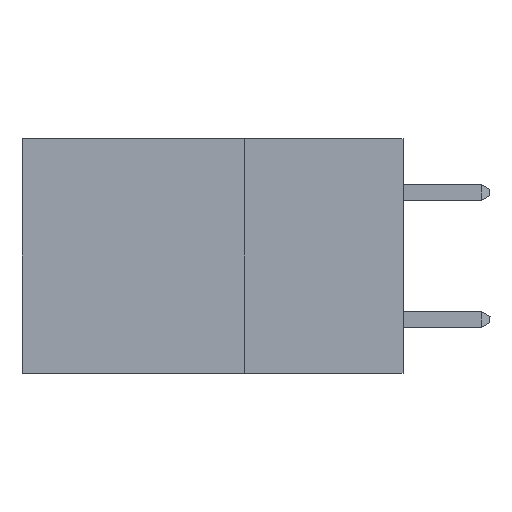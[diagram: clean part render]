
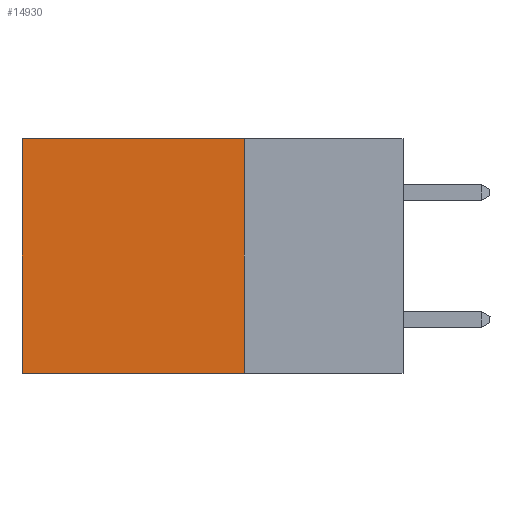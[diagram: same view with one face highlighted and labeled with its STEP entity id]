
A CAD part, left-side view. The second image highlights one B-rep face of the part: STEP entity #14930.
In plain terms, the highlighted planar face has unit normal (-1, 0, 0).
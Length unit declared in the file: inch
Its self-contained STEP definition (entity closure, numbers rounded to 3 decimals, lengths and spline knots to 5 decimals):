
#1055 = ORIENTED_EDGE ( 'NONE', *, *, #9897, .T. ) ;
#1921 = CARTESIAN_POINT ( 'NONE',  ( 0.2875, 0.25, -0.37 ) ) ;
#2106 = DIRECTION ( 'NONE',  ( 0., 0., -1. ) ) ;
#3233 = CARTESIAN_POINT ( 'NONE',  ( 0.2875, 0.25, -0.37 ) ) ;
#3440 = CARTESIAN_POINT ( 'NONE',  ( 0.2875, 0.25, 0. ) ) ;
#4289 = ORIENTED_EDGE ( 'NONE', *, *, #8579, .T. ) ;
#5128 = FACE_OUTER_BOUND ( 'NONE', #14606, .T. ) ;
#6759 = CARTESIAN_POINT ( 'NONE',  ( 0.2875, 0.6, 0. ) ) ;
#8153 = LINE ( 'NONE', #9951, #15845 ) ;
#8352 = CARTESIAN_POINT ( 'NONE',  ( 0.2875, 0.6, -0.37 ) ) ;
#8579 = EDGE_CURVE ( 'NONE', #10266, #15708, #15592, .T. ) ;
#9590 = CARTESIAN_POINT ( 'NONE',  ( 0.2875, 0.6, 0. ) ) ;
#9897 = EDGE_CURVE ( 'NONE', #15708, #12818, #10038, .T. ) ;
#9951 = CARTESIAN_POINT ( 'NONE',  ( 0.2875, 0.25, 0. ) ) ;
#10038 = LINE ( 'NONE', #6759, #16813 ) ;
#10266 = VERTEX_POINT ( 'NONE', #19987 ) ;
#10325 = DIRECTION ( 'NONE',  ( 0., 0., -1. ) ) ;
#10380 = EDGE_CURVE ( 'NONE', #12661, #12818, #18739, .T. ) ;
#10491 = CARTESIAN_POINT ( 'NONE',  ( 0.2875, 0.25, 0. ) ) ;
#10594 = DIRECTION ( 'NONE',  ( 0., 1., 0. ) ) ;
#11295 = EDGE_CURVE ( 'NONE', #10266, #12661, #8153, .T. ) ;
#11465 = VECTOR ( 'NONE', #10594, 39.37008 ) ;
#12015 = PLANE ( 'NONE',  #18959 ) ;
#12661 = VERTEX_POINT ( 'NONE', #1921 ) ;
#12818 = VERTEX_POINT ( 'NONE', #8352 ) ;
#14606 = EDGE_LOOP ( 'NONE', ( #1055, #20991, #22138, #4289 ) ) ;
#14930 = ADVANCED_FACE ( 'NONE', ( #5128 ), #12015, .F. ) ;
#15592 = LINE ( 'NONE', #10491, #11465 ) ;
#15708 = VERTEX_POINT ( 'NONE', #9590 ) ;
#15845 = VECTOR ( 'NONE', #16538, 39.37008 ) ;
#16538 = DIRECTION ( 'NONE',  ( 0., 0., -1. ) ) ;
#16813 = VECTOR ( 'NONE', #2106, 39.37008 ) ;
#16934 = DIRECTION ( 'NONE',  ( 1., 0., 0. ) ) ;
#17847 = VECTOR ( 'NONE', #20224, 39.37008 ) ;
#18739 = LINE ( 'NONE', #3233, #17847 ) ;
#18959 = AXIS2_PLACEMENT_3D ( 'NONE', #3440, #16934, #10325 ) ;
#19987 = CARTESIAN_POINT ( 'NONE',  ( 0.2875, 0.25, 0. ) ) ;
#20224 = DIRECTION ( 'NONE',  ( 0., 1., 0. ) ) ;
#20991 = ORIENTED_EDGE ( 'NONE', *, *, #10380, .F. ) ;
#22138 = ORIENTED_EDGE ( 'NONE', *, *, #11295, .F. ) ;
